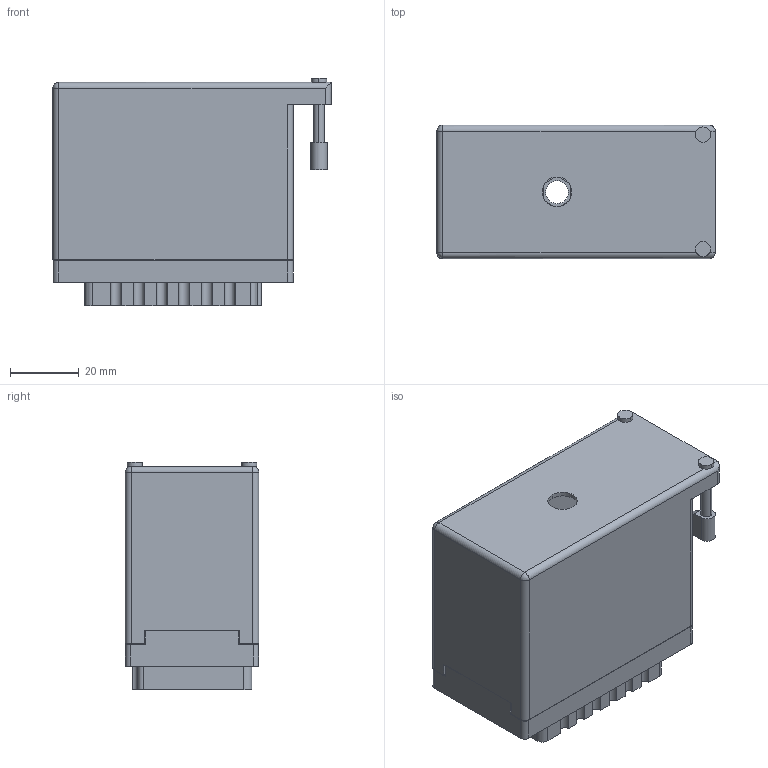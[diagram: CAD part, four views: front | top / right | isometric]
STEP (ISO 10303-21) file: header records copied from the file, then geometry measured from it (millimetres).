
FILE_DESCRIPTION (( 'STEP AP203' ), '1' );
FILE_NAME ('516-120-000-250.STEP', '2020-03-06T23:41:56', ( '' ), ( '' ), 'SwSTEP 2.0', 'SolidWorks 2016', '' );
FILE_SCHEMA (( 'CONFIG_CONTROL_DESIGN' ));
Products named in the file (3): 516 Part Receptacle_120; 516-230-001_Metal - 120 Side Entry; 516-120-000-250
Assembly tree (2 placements, depth 2):
  516-120-000-250
    516 Part Receptacle_120
    516-230-001_Metal - 120 Side Entry
Bounding box: 81.03 x 38.86 x 66.32 mm (x, y, z)
Volume: 43025.1 mm3; surface area: 65138.9 mm2
Topology: 2 solids, 2 shells, 2551 faces, 7582 edges, 5048 vertices
Faces by surface type: plane 1825, cylinder 722, cone 2, sphere 2
Entity records: 86393 total; most frequent: CARTESIAN_POINT 15222, ORIENTED_EDGE 15160, DIRECTION 14610, EDGE_CURVE 7580, LINE 5650, VECTOR 5650, VERTEX_POINT 5048, AXIS2_PLACEMENT_3D 4480
